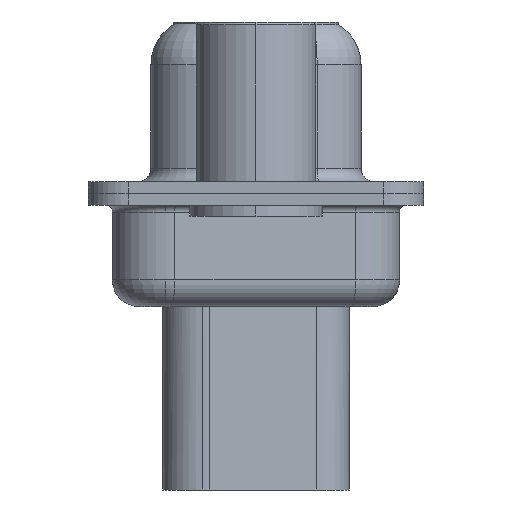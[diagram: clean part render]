
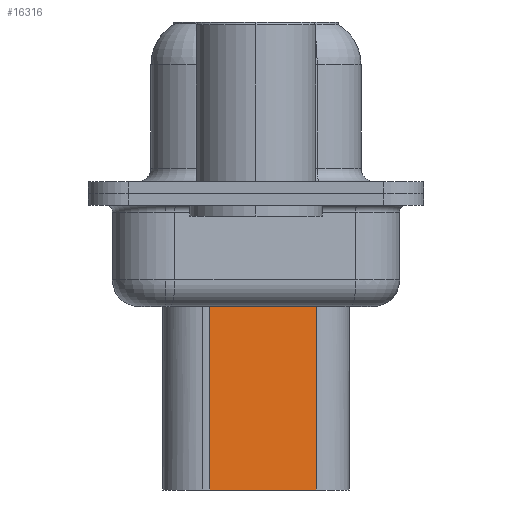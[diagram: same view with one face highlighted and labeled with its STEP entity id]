
A CAD part, left-side view. The second image highlights one B-rep face of the part: STEP entity #16316.
In plain terms, the highlighted planar face has unit normal (-0.985, -0.174, 0).
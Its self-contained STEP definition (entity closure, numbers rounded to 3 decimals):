
#357 = CARTESIAN_POINT ( 'NONE',  ( 5.229, -2.26, -11.15 ) ) ;
#636 = DIRECTION ( 'NONE',  ( -0.174, 0.985, 0. ) ) ;
#1017 = PLANE ( 'NONE',  #17374 ) ;
#2144 = VERTEX_POINT ( 'NONE', #357 ) ;
#2640 = ORIENTED_EDGE ( 'NONE', *, *, #14813, .F. ) ;
#4296 = VECTOR ( 'NONE', #11561, 1000. ) ;
#5929 = CARTESIAN_POINT ( 'NONE',  ( 4.524, 1.74, -11.15 ) ) ;
#6674 = VECTOR ( 'NONE', #15688, 1000. ) ;
#6930 = CARTESIAN_POINT ( 'NONE',  ( 4.524, 1.74, -3.1 ) ) ;
#7374 = CARTESIAN_POINT ( 'NONE',  ( 4.524, 1.74, -3.975 ) ) ;
#7471 = EDGE_CURVE ( 'NONE', #17238, #14037, #15306, .T. ) ;
#8457 = CARTESIAN_POINT ( 'NONE',  ( 4.524, 1.74, -3.1 ) ) ;
#9785 = CARTESIAN_POINT ( 'NONE',  ( 4.524, 1.74, -11.15 ) ) ;
#9829 = VERTEX_POINT ( 'NONE', #5929 ) ;
#10134 = DIRECTION ( 'NONE',  ( 0., 0., -1. ) ) ;
#10162 = EDGE_CURVE ( 'NONE', #14037, #9829, #12945, .T. ) ;
#11257 = LINE ( 'NONE', #9785, #6674 ) ;
#11458 = DIRECTION ( 'NONE',  ( 0.174, -0.985, 0. ) ) ;
#11561 = DIRECTION ( 'NONE',  ( 0., 0., -1. ) ) ;
#11639 = EDGE_LOOP ( 'NONE', ( #2640, #15611, #17968, #12962 ) ) ;
#11654 = VECTOR ( 'NONE', #636, 1000. ) ;
#12945 = LINE ( 'NONE', #8457, #17002 ) ;
#12962 = ORIENTED_EDGE ( 'NONE', *, *, #17569, .F. ) ;
#13188 = LINE ( 'NONE', #13286, #4296 ) ;
#13286 = CARTESIAN_POINT ( 'NONE',  ( 5.229, -2.26, -3.1 ) ) ;
#13972 = CARTESIAN_POINT ( 'NONE',  ( 4.353, 2.709, -3.975 ) ) ;
#14037 = VERTEX_POINT ( 'NONE', #7374 ) ;
#14813 = EDGE_CURVE ( 'NONE', #17238, #2144, #13188, .T. ) ;
#15306 = LINE ( 'NONE', #13972, #11654 ) ;
#15611 = ORIENTED_EDGE ( 'NONE', *, *, #7471, .T. ) ;
#15688 = DIRECTION ( 'NONE',  ( -0.174, 0.985, 0. ) ) ;
#15914 = CARTESIAN_POINT ( 'NONE',  ( 5.229, -2.26, -3.975 ) ) ;
#15976 = DIRECTION ( 'NONE',  ( -0.985, -0.174, 0. ) ) ;
#16084 = FACE_OUTER_BOUND ( 'NONE', #11639, .T. ) ;
#16316 = ADVANCED_FACE ( 'NONE', ( #16084 ), #1017, .T. ) ;
#17002 = VECTOR ( 'NONE', #10134, 1000. ) ;
#17238 = VERTEX_POINT ( 'NONE', #15914 ) ;
#17374 = AXIS2_PLACEMENT_3D ( 'NONE', #6930, #15976, #11458 ) ;
#17569 = EDGE_CURVE ( 'NONE', #2144, #9829, #11257, .T. ) ;
#17968 = ORIENTED_EDGE ( 'NONE', *, *, #10162, .T. ) ;
